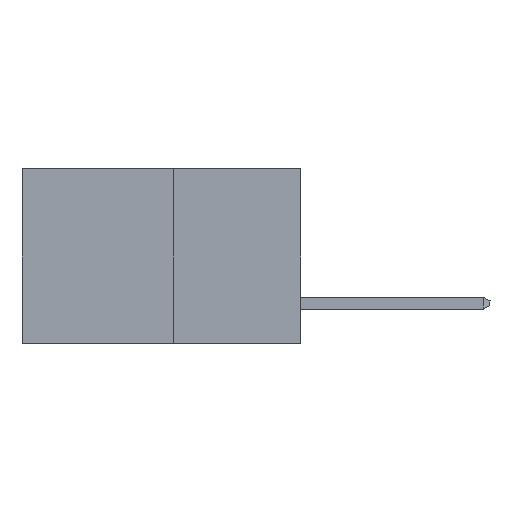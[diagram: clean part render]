
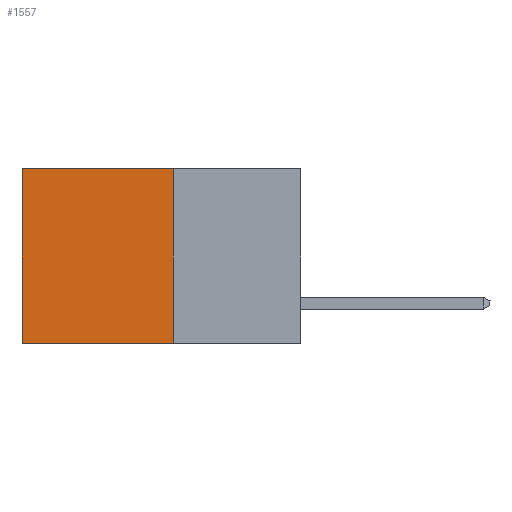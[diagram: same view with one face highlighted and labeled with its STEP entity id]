
A CAD part, left-side view. The second image highlights one B-rep face of the part: STEP entity #1557.
In plain terms, the highlighted planar face has unit normal (-1, 0, 0).
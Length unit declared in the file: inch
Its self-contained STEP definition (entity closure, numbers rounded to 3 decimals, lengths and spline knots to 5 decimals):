
#44 = EDGE_CURVE ( 'NONE', #5576, #6766, #3991, .T. ) ;
#240 = EDGE_CURVE ( 'NONE', #6766, #7318, #7854, .T. ) ;
#405 = ORIENTED_EDGE ( 'NONE', *, *, #240, .T. ) ;
#644 = CARTESIAN_POINT ( 'NONE',  ( 0.277, 0.27, 0. ) ) ;
#980 = ORIENTED_EDGE ( 'NONE', *, *, #44, .T. ) ;
#1557 = ADVANCED_FACE ( 'NONE', ( #4236 ), #10126, .F. ) ;
#1682 = CARTESIAN_POINT ( 'NONE',  ( 0.277, 0.27, 0. ) ) ;
#2296 = EDGE_CURVE ( 'NONE', #7465, #7318, #4482, .T. ) ;
#2573 = LINE ( 'NONE', #6751, #8559 ) ;
#2746 = DIRECTION ( 'NONE',  ( 1., 0., 0. ) ) ;
#2837 = EDGE_CURVE ( 'NONE', #5576, #7465, #2573, .T. ) ;
#2945 = DIRECTION ( 'NONE',  ( 0., 1., 0. ) ) ;
#3283 = CARTESIAN_POINT ( 'NONE',  ( 0.277, 0.27, -0.37 ) ) ;
#3657 = EDGE_LOOP ( 'NONE', ( #405, #5425, #7352, #980 ) ) ;
#3991 = LINE ( 'NONE', #1682, #5942 ) ;
#4236 = FACE_OUTER_BOUND ( 'NONE', #3657, .T. ) ;
#4482 = LINE ( 'NONE', #3283, #10103 ) ;
#4601 = CARTESIAN_POINT ( 'NONE',  ( 0.277, 0.27, -0.37 ) ) ;
#4677 = AXIS2_PLACEMENT_3D ( 'NONE', #4601, #2746, #10102 ) ;
#5425 = ORIENTED_EDGE ( 'NONE', *, *, #2296, .F. ) ;
#5450 = CARTESIAN_POINT ( 'NONE',  ( 0.277, 0.27, -0.37 ) ) ;
#5576 = VERTEX_POINT ( 'NONE', #644 ) ;
#5942 = VECTOR ( 'NONE', #2945, 39.37008 ) ;
#6072 = VECTOR ( 'NONE', #9950, 39.37008 ) ;
#6210 = CARTESIAN_POINT ( 'NONE',  ( 0.277, 0.59, -0.37 ) ) ;
#6751 = CARTESIAN_POINT ( 'NONE',  ( 0.277, 0.27, -0.37 ) ) ;
#6766 = VERTEX_POINT ( 'NONE', #6781 ) ;
#6778 = DIRECTION ( 'NONE',  ( 0., 1., 0. ) ) ;
#6781 = CARTESIAN_POINT ( 'NONE',  ( 0.277, 0.59, 0. ) ) ;
#6827 = DIRECTION ( 'NONE',  ( 0., 0., -1. ) ) ;
#7318 = VERTEX_POINT ( 'NONE', #6210 ) ;
#7352 = ORIENTED_EDGE ( 'NONE', *, *, #2837, .F. ) ;
#7465 = VERTEX_POINT ( 'NONE', #5450 ) ;
#7854 = LINE ( 'NONE', #9862, #6072 ) ;
#8559 = VECTOR ( 'NONE', #6827, 39.37008 ) ;
#9862 = CARTESIAN_POINT ( 'NONE',  ( 0.277, 0.59, -0.37 ) ) ;
#9950 = DIRECTION ( 'NONE',  ( 0., 0., -1. ) ) ;
#10102 = DIRECTION ( 'NONE',  ( 0., 0., -1. ) ) ;
#10103 = VECTOR ( 'NONE', #6778, 39.37008 ) ;
#10126 = PLANE ( 'NONE',  #4677 ) ;
